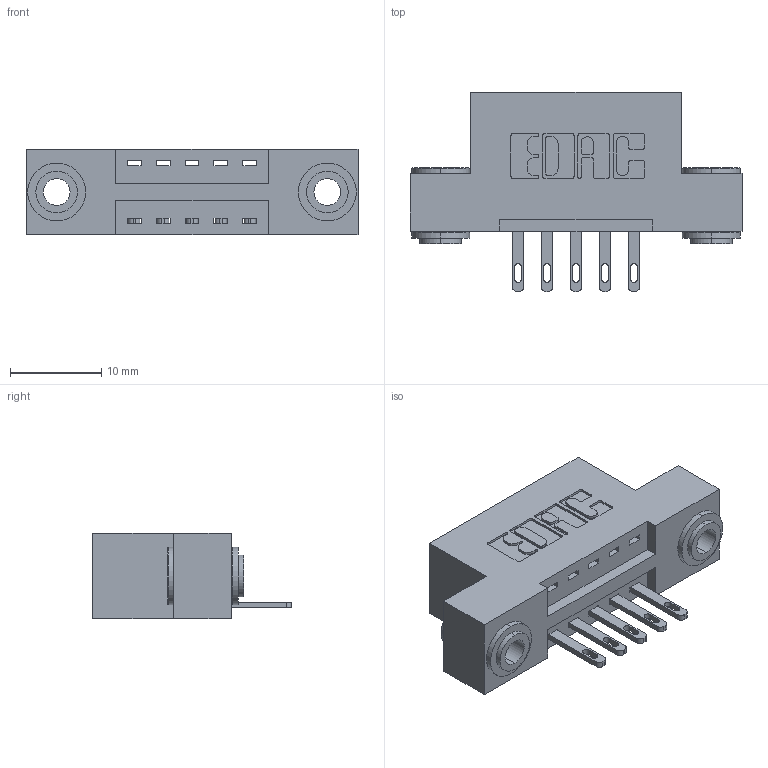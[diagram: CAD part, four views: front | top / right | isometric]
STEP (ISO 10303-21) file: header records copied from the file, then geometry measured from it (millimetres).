
FILE_DESCRIPTION (( 'STEP AP203' ), '1' );
FILE_NAME ('346-005-500-103.STEP', '2022-05-04T17:18:05', ( '' ), ( '' ), 'SwSTEP 2.0', 'SolidWorks 2020', '' );
FILE_SCHEMA (( 'CONFIG_CONTROL_DESIGN' ));
Length unit declared in the file: inch
Products named in the file (4): 346-005-500-103; 345-292-001_345-293-100; 345-250-002_345-250-002-102; 346 Part_Flush Mounting Lugs - 0.156 Dia-TH
Assembly tree (8 placements, depth 2):
  346-005-500-103
    346 Part_Flush Mounting Lugs - 0.156 Dia-TH
    345-292-001_345-293-100  x5
    345-250-002_345-250-002-102  x2
Bounding box: 36.45 x 21.84 x 9.4 mm (x, y, z)
Volume: 3238.4 mm3; surface area: 3911.5 mm2
Topology: 8 solids, 8 shells, 444 faces, 1281 edges, 850 vertices
Faces by surface type: plane 270, cylinder 166, cone 8
Entity records: 9080 total; most frequent: CARTESIAN_POINT 1548, ORIENTED_EDGE 1478, DIRECTION 1443, EDGE_CURVE 739, VECTOR 559, LINE 559, VERTEX_POINT 490, AXIS2_PLACEMENT_3D 442
